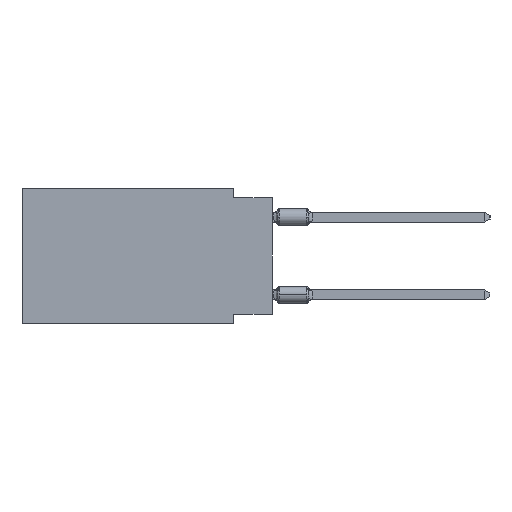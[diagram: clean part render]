
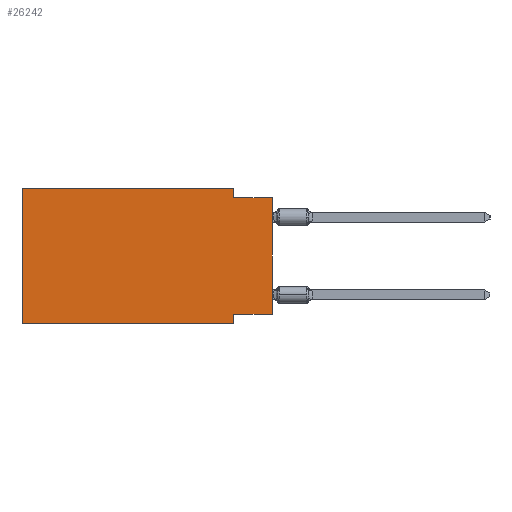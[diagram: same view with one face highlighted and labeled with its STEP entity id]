
A CAD part, left-side view. The second image highlights one B-rep face of the part: STEP entity #26242.
In plain terms, the highlighted planar face has unit normal (-1, 0, 0).
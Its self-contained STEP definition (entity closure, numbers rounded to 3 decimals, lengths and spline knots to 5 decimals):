
#359 = CARTESIAN_POINT ( 'NONE',  ( 0., 0.1, -0.025 ) ) ;
#2320 = CARTESIAN_POINT ( 'NONE',  ( 0., 0.645, -0.35 ) ) ;
#2646 = DIRECTION ( 'NONE',  ( 0., -1., 0. ) ) ;
#3036 = DIRECTION ( 'NONE',  ( 0., 0., -1. ) ) ;
#3951 = DIRECTION ( 'NONE',  ( 0., 0., 1. ) ) ;
#3968 = CARTESIAN_POINT ( 'NONE',  ( 0., 0., -0.325 ) ) ;
#5409 = VERTEX_POINT ( 'NONE', #38783 ) ;
#7575 = DIRECTION ( 'NONE',  ( 1., 0., 0. ) ) ;
#7593 = VERTEX_POINT ( 'NONE', #27738 ) ;
#7920 = LINE ( 'NONE', #27341, #40121 ) ;
#10087 = VECTOR ( 'NONE', #17675, 39.37008 ) ;
#10605 = EDGE_CURVE ( 'NONE', #59726, #5409, #41958, .T. ) ;
#11159 = VECTOR ( 'NONE', #52089, 39.37008 ) ;
#11715 = CARTESIAN_POINT ( 'NONE',  ( 0., 0.645, 0. ) ) ;
#12468 = ORIENTED_EDGE ( 'NONE', *, *, #45875, .F. ) ;
#13061 = CARTESIAN_POINT ( 'NONE',  ( 0., 0.1, -0.35 ) ) ;
#16323 = LINE ( 'NONE', #26842, #26858 ) ;
#17164 = EDGE_CURVE ( 'NONE', #23545, #7593, #47940, .T. ) ;
#17675 = DIRECTION ( 'NONE',  ( 0., 0., 1. ) ) ;
#18250 = CARTESIAN_POINT ( 'NONE',  ( 0., 0.645, 0. ) ) ;
#18817 = ORIENTED_EDGE ( 'NONE', *, *, #10605, .T. ) ;
#19169 = ORIENTED_EDGE ( 'NONE', *, *, #62406, .F. ) ;
#19543 = VERTEX_POINT ( 'NONE', #56125 ) ;
#20467 = DIRECTION ( 'NONE',  ( 0., -1., 0. ) ) ;
#21366 = AXIS2_PLACEMENT_3D ( 'NONE', #11715, #7575, #41061 ) ;
#21789 = VECTOR ( 'NONE', #3951, 39.37008 ) ;
#23213 = ORIENTED_EDGE ( 'NONE', *, *, #17164, .F. ) ;
#23545 = VERTEX_POINT ( 'NONE', #2320 ) ;
#23809 = VERTEX_POINT ( 'NONE', #359 ) ;
#24362 = VERTEX_POINT ( 'NONE', #35617 ) ;
#24634 = ORIENTED_EDGE ( 'NONE', *, *, #52115, .T. ) ;
#26242 = ADVANCED_FACE ( 'NONE', ( #55406 ), #45233, .F. ) ;
#26842 = CARTESIAN_POINT ( 'NONE',  ( 0., 0., -0.025 ) ) ;
#26858 = VECTOR ( 'NONE', #20467, 39.37008 ) ;
#27341 = CARTESIAN_POINT ( 'NONE',  ( 0., 0.645, 0. ) ) ;
#27738 = CARTESIAN_POINT ( 'NONE',  ( 0., 0.645, 0. ) ) ;
#35617 = CARTESIAN_POINT ( 'NONE',  ( 0., 0.1, -0.325 ) ) ;
#36417 = LINE ( 'NONE', #55870, #51435 ) ;
#36685 = DIRECTION ( 'NONE',  ( 0., 0., -1. ) ) ;
#38050 = LINE ( 'NONE', #3968, #11159 ) ;
#38525 = EDGE_CURVE ( 'NONE', #59726, #24362, #38050, .T. ) ;
#38783 = CARTESIAN_POINT ( 'NONE',  ( 0., 0., -0.025 ) ) ;
#38936 = VECTOR ( 'NONE', #3036, 39.37008 ) ;
#40121 = VECTOR ( 'NONE', #41099, 39.37008 ) ;
#41061 = DIRECTION ( 'NONE',  ( 0., 0., -1. ) ) ;
#41099 = DIRECTION ( 'NONE',  ( 0., -1., 0. ) ) ;
#41624 = CARTESIAN_POINT ( 'NONE',  ( 0., 0.1, 0. ) ) ;
#41693 = EDGE_CURVE ( 'NONE', #19543, #23809, #56262, .T. ) ;
#41958 = LINE ( 'NONE', #61383, #10087 ) ;
#43223 = EDGE_CURVE ( 'NONE', #23809, #5409, #16323, .T. ) ;
#44283 = VECTOR ( 'NONE', #36685, 39.37008 ) ;
#45233 = PLANE ( 'NONE',  #21366 ) ;
#45875 = EDGE_CURVE ( 'NONE', #24362, #47950, #51660, .T. ) ;
#47940 = LINE ( 'NONE', #18250, #21789 ) ;
#47950 = VERTEX_POINT ( 'NONE', #61708 ) ;
#51435 = VECTOR ( 'NONE', #2646, 39.37008 ) ;
#51660 = LINE ( 'NONE', #13061, #44283 ) ;
#52089 = DIRECTION ( 'NONE',  ( 0., 1., 0. ) ) ;
#52115 = EDGE_CURVE ( 'NONE', #23545, #47950, #36417, .T. ) ;
#53779 = ORIENTED_EDGE ( 'NONE', *, *, #38525, .F. ) ;
#55406 = FACE_OUTER_BOUND ( 'NONE', #60907, .T. ) ;
#55870 = CARTESIAN_POINT ( 'NONE',  ( 0., 0.645, -0.35 ) ) ;
#56125 = CARTESIAN_POINT ( 'NONE',  ( 0., 0.1, 0. ) ) ;
#56262 = LINE ( 'NONE', #41624, #38936 ) ;
#57943 = CARTESIAN_POINT ( 'NONE',  ( 0., 0., -0.325 ) ) ;
#59440 = ORIENTED_EDGE ( 'NONE', *, *, #41693, .F. ) ;
#59726 = VERTEX_POINT ( 'NONE', #57943 ) ;
#60907 = EDGE_LOOP ( 'NONE', ( #18817, #62921, #59440, #19169, #23213, #24634, #12468, #53779 ) ) ;
#61383 = CARTESIAN_POINT ( 'NONE',  ( 0., 0., 0. ) ) ;
#61708 = CARTESIAN_POINT ( 'NONE',  ( 0., 0.1, -0.35 ) ) ;
#62406 = EDGE_CURVE ( 'NONE', #7593, #19543, #7920, .T. ) ;
#62921 = ORIENTED_EDGE ( 'NONE', *, *, #43223, .F. ) ;
